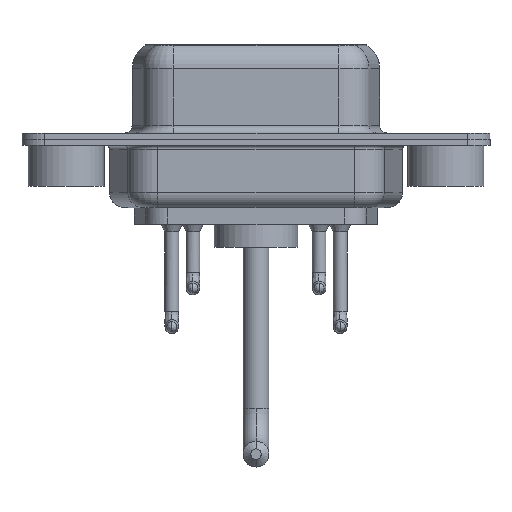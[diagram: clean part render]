
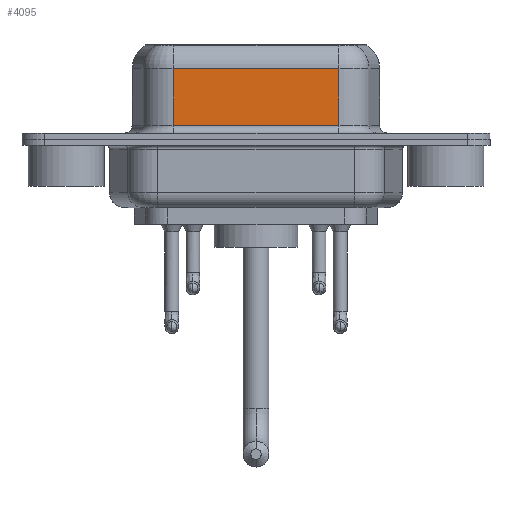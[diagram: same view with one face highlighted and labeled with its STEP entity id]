
A CAD part, front view. The second image highlights one B-rep face of the part: STEP entity #4095.
In plain terms, the highlighted planar face has unit normal (0, -1, 0).
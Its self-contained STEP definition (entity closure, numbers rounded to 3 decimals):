
#312 = FACE_OUTER_BOUND ( 'NONE', #4776, .T. ) ;
#444 = CARTESIAN_POINT ( 'NONE',  ( 7.038, -3.95, 4.65 ) ) ;
#1048 = CARTESIAN_POINT ( 'NONE',  ( 17.962, -3.95, 6.4 ) ) ;
#1178 = AXIS2_PLACEMENT_3D ( 'NONE', #3840, #8876, #9117 ) ;
#1200 = ORIENTED_EDGE ( 'NONE', *, *, #13024, .T. ) ;
#1638 = EDGE_CURVE ( 'NONE', #15906, #15333, #2771, .T. ) ;
#1657 = VECTOR ( 'NONE', #13445, 1000. ) ;
#2600 = EDGE_CURVE ( 'NONE', #5682, #15333, #15936, .T. ) ;
#2771 = LINE ( 'NONE', #12002, #4839 ) ;
#2779 = PLANE ( 'NONE',  #1178 ) ;
#3840 = CARTESIAN_POINT ( 'NONE',  ( 17.962, -3.95, 6.4 ) ) ;
#4095 = ADVANCED_FACE ( 'NONE', ( #312 ), #2779, .F. ) ;
#4776 = EDGE_LOOP ( 'NONE', ( #12306, #6376, #1200, #12808 ) ) ;
#4839 = VECTOR ( 'NONE', #11915, 1000. ) ;
#5318 = LINE ( 'NONE', #11772, #16204 ) ;
#5448 = CARTESIAN_POINT ( 'NONE',  ( 17.962, -3.95, 4.65 ) ) ;
#5682 = VERTEX_POINT ( 'NONE', #5448 ) ;
#6321 = CARTESIAN_POINT ( 'NONE',  ( 17.962, -3.95, 0.9 ) ) ;
#6376 = ORIENTED_EDGE ( 'NONE', *, *, #15498, .T. ) ;
#6644 = DIRECTION ( 'NONE',  ( -1., 0., 0. ) ) ;
#6859 = CARTESIAN_POINT ( 'NONE',  ( 7.038, -3.95, 0.9 ) ) ;
#7388 = VERTEX_POINT ( 'NONE', #444 ) ;
#8876 = DIRECTION ( 'NONE',  ( 0., 1., 0. ) ) ;
#9117 = DIRECTION ( 'NONE',  ( -1., 0., 0. ) ) ;
#9757 = DIRECTION ( 'NONE',  ( 0., 0., -1. ) ) ;
#11011 = CARTESIAN_POINT ( 'NONE',  ( 7.038, -3.95, 6.4 ) ) ;
#11638 = VECTOR ( 'NONE', #9757, 1000. ) ;
#11772 = CARTESIAN_POINT ( 'NONE',  ( 17.962, -3.95, 4.65 ) ) ;
#11915 = DIRECTION ( 'NONE',  ( 1., 0., 0. ) ) ;
#12002 = CARTESIAN_POINT ( 'NONE',  ( 17.962, -3.95, 0.9 ) ) ;
#12306 = ORIENTED_EDGE ( 'NONE', *, *, #2600, .F. ) ;
#12808 = ORIENTED_EDGE ( 'NONE', *, *, #1638, .T. ) ;
#13024 = EDGE_CURVE ( 'NONE', #7388, #15906, #16167, .T. ) ;
#13445 = DIRECTION ( 'NONE',  ( 0., 0., -1. ) ) ;
#15333 = VERTEX_POINT ( 'NONE', #6321 ) ;
#15498 = EDGE_CURVE ( 'NONE', #5682, #7388, #5318, .T. ) ;
#15906 = VERTEX_POINT ( 'NONE', #6859 ) ;
#15936 = LINE ( 'NONE', #1048, #1657 ) ;
#16167 = LINE ( 'NONE', #11011, #11638 ) ;
#16204 = VECTOR ( 'NONE', #6644, 1000. ) ;
